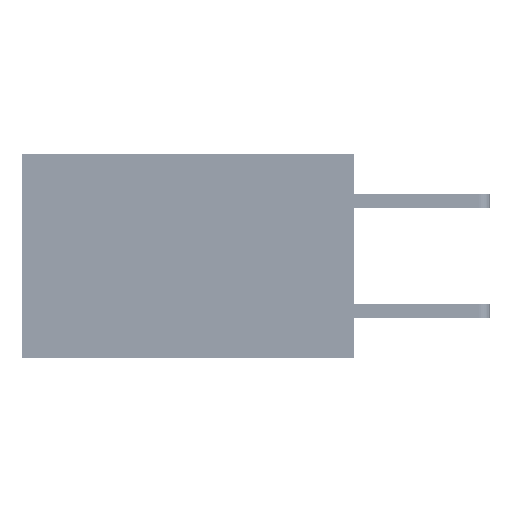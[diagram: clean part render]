
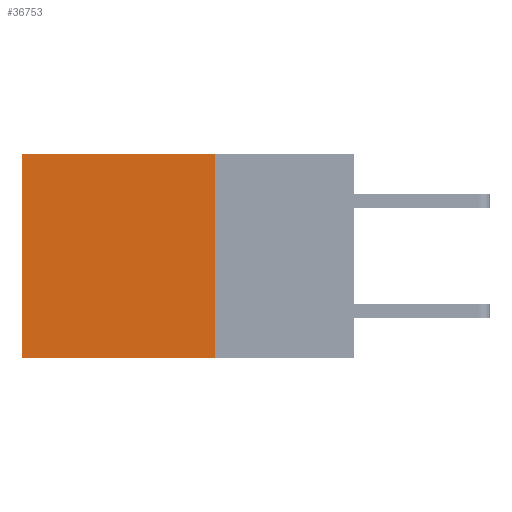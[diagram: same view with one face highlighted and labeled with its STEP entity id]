
A CAD part, left-side view. The second image highlights one B-rep face of the part: STEP entity #36753.
In plain terms, the highlighted planar face has unit normal (-1, 0, 0).
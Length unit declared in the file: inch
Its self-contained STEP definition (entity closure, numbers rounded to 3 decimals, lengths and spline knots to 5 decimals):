
#383 = DIRECTION ( 'NONE',  ( 1., 0., 0. ) ) ;
#692 = EDGE_CURVE ( 'NONE', #35913, #19282, #37731, .T. ) ;
#1664 = ORIENTED_EDGE ( 'NONE', *, *, #20856, .F. ) ;
#2999 = CARTESIAN_POINT ( 'NONE',  ( 0.2875, 0.25, 0. ) ) ;
#3978 = DIRECTION ( 'NONE',  ( 0., 1., 0. ) ) ;
#4456 = LINE ( 'NONE', #12254, #31274 ) ;
#5194 = ORIENTED_EDGE ( 'NONE', *, *, #43556, .T. ) ;
#5745 = ORIENTED_EDGE ( 'NONE', *, *, #692, .T. ) ;
#5908 = VERTEX_POINT ( 'NONE', #9862 ) ;
#6500 = ORIENTED_EDGE ( 'NONE', *, *, #26026, .F. ) ;
#7931 = FACE_OUTER_BOUND ( 'NONE', #24755, .T. ) ;
#8065 = CARTESIAN_POINT ( 'NONE',  ( 0.2875, 0.6, 0. ) ) ;
#8301 = AXIS2_PLACEMENT_3D ( 'NONE', #12444, #383, #46687 ) ;
#9862 = CARTESIAN_POINT ( 'NONE',  ( 0.2875, 0.6, -0.37 ) ) ;
#10137 = CARTESIAN_POINT ( 'NONE',  ( 0.2875, 0.6, 0. ) ) ;
#10304 = DIRECTION ( 'NONE',  ( 0., 1., 0. ) ) ;
#12254 = CARTESIAN_POINT ( 'NONE',  ( 0.2875, 0.25, -0.37 ) ) ;
#12444 = CARTESIAN_POINT ( 'NONE',  ( 0.2875, 0.25, 0. ) ) ;
#16279 = CARTESIAN_POINT ( 'NONE',  ( 0.2875, 0.25, -0.37 ) ) ;
#17945 = DIRECTION ( 'NONE',  ( 0., 0., -1. ) ) ;
#19282 = VERTEX_POINT ( 'NONE', #8065 ) ;
#20856 = EDGE_CURVE ( 'NONE', #27765, #5908, #4456, .T. ) ;
#21543 = VECTOR ( 'NONE', #17945, 39.37008 ) ;
#24755 = EDGE_LOOP ( 'NONE', ( #5194, #1664, #6500, #5745 ) ) ;
#25671 = DIRECTION ( 'NONE',  ( 0., 0., -1. ) ) ;
#26026 = EDGE_CURVE ( 'NONE', #35913, #27765, #36974, .T. ) ;
#27765 = VERTEX_POINT ( 'NONE', #16279 ) ;
#31274 = VECTOR ( 'NONE', #3978, 39.37008 ) ;
#33404 = VECTOR ( 'NONE', #25671, 39.37008 ) ;
#35363 = PLANE ( 'NONE',  #8301 ) ;
#35913 = VERTEX_POINT ( 'NONE', #46626 ) ;
#36753 = ADVANCED_FACE ( 'NONE', ( #7931 ), #35363, .F. ) ;
#36974 = LINE ( 'NONE', #2999, #33404 ) ;
#37731 = LINE ( 'NONE', #44804, #42244 ) ;
#40356 = LINE ( 'NONE', #10137, #21543 ) ;
#42244 = VECTOR ( 'NONE', #10304, 39.37008 ) ;
#43556 = EDGE_CURVE ( 'NONE', #19282, #5908, #40356, .T. ) ;
#44804 = CARTESIAN_POINT ( 'NONE',  ( 0.2875, 0.25, 0. ) ) ;
#46626 = CARTESIAN_POINT ( 'NONE',  ( 0.2875, 0.25, 0. ) ) ;
#46687 = DIRECTION ( 'NONE',  ( 0., 0., -1. ) ) ;
